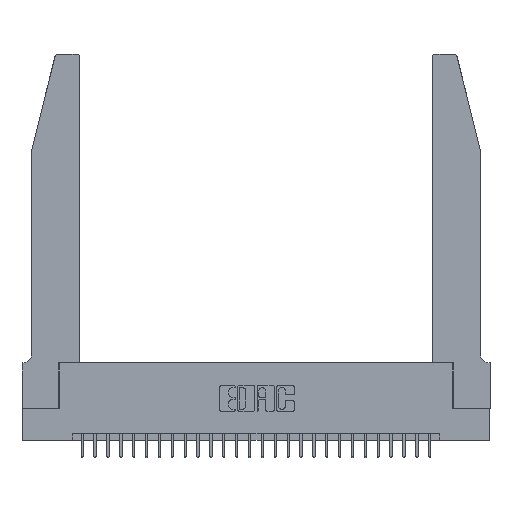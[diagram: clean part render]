
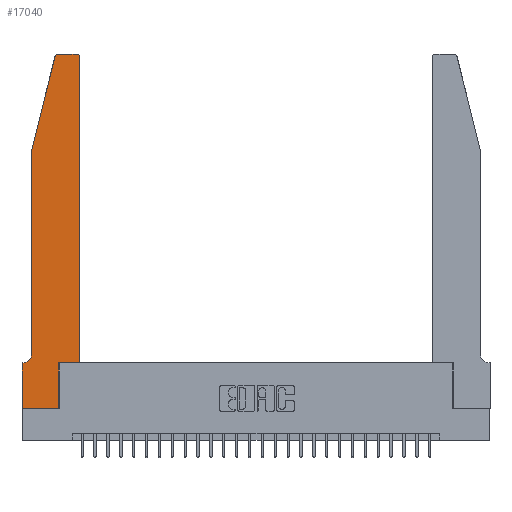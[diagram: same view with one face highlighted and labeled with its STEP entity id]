
A CAD part, top view. The second image highlights one B-rep face of the part: STEP entity #17040.
In plain terms, the highlighted planar face has unit normal (0, 0, 1).
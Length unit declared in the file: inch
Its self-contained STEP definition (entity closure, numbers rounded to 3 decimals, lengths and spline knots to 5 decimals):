
#171 = EDGE_CURVE ( 'NONE', #16835, #24822, #9577, .T. ) ;
#645 = EDGE_CURVE ( 'NONE', #26955, #16835, #19283, .T. ) ;
#752 = LINE ( 'NONE', #22707, #5583 ) ;
#1592 = VERTEX_POINT ( 'NONE', #20082 ) ;
#1924 = CARTESIAN_POINT ( 'NONE',  ( 0., 0.35, 0.37 ) ) ;
#1952 = ORIENTED_EDGE ( 'NONE', *, *, #23661, .T. ) ;
#2432 = ORIENTED_EDGE ( 'NONE', *, *, #6540, .T. ) ;
#2747 = CARTESIAN_POINT ( 'NONE',  ( 0.0755, 2., 0.37 ) ) ;
#3024 = DIRECTION ( 'NONE',  ( 0., 1., 0. ) ) ;
#3047 = LINE ( 'NONE', #7139, #26902 ) ;
#3070 = VECTOR ( 'NONE', #17211, 39.37008 ) ;
#3137 = EDGE_CURVE ( 'NONE', #22423, #17642, #752, .T. ) ;
#3469 = EDGE_LOOP ( 'NONE', ( #27641, #12043, #7407, #23063, #1952, #2432, #8991, #21217, #19030, #14105, #15593, #9170 ) ) ;
#4006 = CARTESIAN_POINT ( 'NONE',  ( 0.284, 2.72, 0.37 ) ) ;
#4182 = VERTEX_POINT ( 'NONE', #27566 ) ;
#4199 = LINE ( 'NONE', #13072, #23433 ) ;
#4328 = EDGE_CURVE ( 'NONE', #17642, #25782, #17723, .T. ) ;
#4674 = CARTESIAN_POINT ( 'NONE',  ( 0., 0., 0.37 ) ) ;
#4693 = CARTESIAN_POINT ( 'NONE',  ( 0.4205, 2.72, 0.37 ) ) ;
#4817 = CARTESIAN_POINT ( 'NONE',  ( 0.0755, 2., 0.37 ) ) ;
#5359 = DIRECTION ( 'NONE',  ( 0., -1., 0. ) ) ;
#5583 = VECTOR ( 'NONE', #18510, 39.37008 ) ;
#5661 = CARTESIAN_POINT ( 'NONE',  ( 0.2865, 0.35, 0.37 ) ) ;
#5664 = VERTEX_POINT ( 'NONE', #7063 ) ;
#6540 = EDGE_CURVE ( 'NONE', #1592, #5664, #3047, .T. ) ;
#7063 = CARTESIAN_POINT ( 'NONE',  ( 0., 0.35, 0.37 ) ) ;
#7139 = CARTESIAN_POINT ( 'NONE',  ( 0.0755, 0.35, 0.37 ) ) ;
#7407 = ORIENTED_EDGE ( 'NONE', *, *, #19415, .T. ) ;
#7457 = CARTESIAN_POINT ( 'NONE',  ( 0.4505, 0.35, 0.37 ) ) ;
#8480 = LINE ( 'NONE', #24032, #3070 ) ;
#8991 = ORIENTED_EDGE ( 'NONE', *, *, #9553, .T. ) ;
#9170 = ORIENTED_EDGE ( 'NONE', *, *, #15286, .T. ) ;
#9180 = DIRECTION ( 'NONE',  ( 0., -1., 0. ) ) ;
#9553 = EDGE_CURVE ( 'NONE', #5664, #13724, #25017, .T. ) ;
#9577 = LINE ( 'NONE', #18894, #24126 ) ;
#10102 = CARTESIAN_POINT ( 'NONE',  ( 0.284, 2.75, 0.37 ) ) ;
#10204 = FACE_OUTER_BOUND ( 'NONE', #3469, .T. ) ;
#10585 = CARTESIAN_POINT ( 'NONE',  ( 0.0755, 0.42, 0.37 ) ) ;
#10708 = DIRECTION ( 'NONE',  ( 1., 0., 0. ) ) ;
#10867 = CARTESIAN_POINT ( 'NONE',  ( 0.0055, 0.42, 0.37 ) ) ;
#10891 = DIRECTION ( 'NONE',  ( 0., 1., 0. ) ) ;
#11003 = VECTOR ( 'NONE', #25019, 39.37008 ) ;
#11468 = CARTESIAN_POINT ( 'NONE',  ( 0., 0., 0.37 ) ) ;
#12043 = ORIENTED_EDGE ( 'NONE', *, *, #4328, .T. ) ;
#12755 = DIRECTION ( 'NONE',  ( 0., 0., -1. ) ) ;
#12779 = VECTOR ( 'NONE', #9180, 39.37008 ) ;
#12880 = DIRECTION ( 'NONE',  ( 0., 0., 1. ) ) ;
#13072 = CARTESIAN_POINT ( 'NONE',  ( 0.2865, 0.35, 0.37 ) ) ;
#13632 = VERTEX_POINT ( 'NONE', #27018 ) ;
#13724 = VERTEX_POINT ( 'NONE', #11468 ) ;
#14105 = ORIENTED_EDGE ( 'NONE', *, *, #645, .T. ) ;
#15121 = CARTESIAN_POINT ( 'NONE',  ( 0.4205, 2.75, 0.37 ) ) ;
#15286 = EDGE_CURVE ( 'NONE', #24822, #22423, #20137, .T. ) ;
#15309 = DIRECTION ( 'NONE',  ( 1., 0., 0. ) ) ;
#15593 = ORIENTED_EDGE ( 'NONE', *, *, #171, .T. ) ;
#16607 = LINE ( 'NONE', #4817, #11003 ) ;
#16835 = VERTEX_POINT ( 'NONE', #7457 ) ;
#16939 = AXIS2_PLACEMENT_3D ( 'NONE', #1924, #19094, #15309 ) ;
#17040 = ADVANCED_FACE ( 'NONE', ( #10204 ), #26178, .T. ) ;
#17211 = DIRECTION ( 'NONE',  ( 1., 0., 0. ) ) ;
#17388 = DIRECTION ( 'NONE',  ( 1., 0., 0. ) ) ;
#17508 = EDGE_CURVE ( 'NONE', #13632, #26955, #4199, .T. ) ;
#17642 = VERTEX_POINT ( 'NONE', #10102 ) ;
#17723 = CIRCLE ( 'NONE', #21889, 0.03 ) ;
#18510 = DIRECTION ( 'NONE',  ( -1., 0., 0. ) ) ;
#18785 = CARTESIAN_POINT ( 'NONE',  ( 0.4505, 2.72, 0.37 ) ) ;
#18894 = CARTESIAN_POINT ( 'NONE',  ( 0.4505, 0.35, 0.37 ) ) ;
#19030 = ORIENTED_EDGE ( 'NONE', *, *, #17508, .T. ) ;
#19094 = DIRECTION ( 'NONE',  ( 0., 0., 1. ) ) ;
#19283 = LINE ( 'NONE', #23491, #23694 ) ;
#19415 = EDGE_CURVE ( 'NONE', #25782, #4182, #16607, .T. ) ;
#20082 = CARTESIAN_POINT ( 'NONE',  ( 0.0055, 0.35, 0.37 ) ) ;
#20137 = CIRCLE ( 'NONE', #20591, 0.03 ) ;
#20466 = DIRECTION ( 'NONE',  ( -1., 0., 0. ) ) ;
#20591 = AXIS2_PLACEMENT_3D ( 'NONE', #4693, #24194, #24330 ) ;
#21217 = ORIENTED_EDGE ( 'NONE', *, *, #25777, .T. ) ;
#21299 = CIRCLE ( 'NONE', #25455, 0.07 ) ;
#21710 = CARTESIAN_POINT ( 'NONE',  ( 0.25487, 2.72718, 0.37 ) ) ;
#21889 = AXIS2_PLACEMENT_3D ( 'NONE', #4006, #12880, #10708 ) ;
#22255 = EDGE_CURVE ( 'NONE', #4182, #26745, #24993, .T. ) ;
#22423 = VERTEX_POINT ( 'NONE', #15121 ) ;
#22707 = CARTESIAN_POINT ( 'NONE',  ( 0.2605, 2.75, 0.37 ) ) ;
#22834 = DIRECTION ( 'NONE',  ( -1., 0., 0. ) ) ;
#23063 = ORIENTED_EDGE ( 'NONE', *, *, #22255, .T. ) ;
#23433 = VECTOR ( 'NONE', #10891, 39.37008 ) ;
#23491 = CARTESIAN_POINT ( 'NONE',  ( 0.4505, 0.35, 0.37 ) ) ;
#23661 = EDGE_CURVE ( 'NONE', #26745, #1592, #21299, .T. ) ;
#23694 = VECTOR ( 'NONE', #17388, 39.37008 ) ;
#24032 = CARTESIAN_POINT ( 'NONE',  ( 0., 0., 0.37 ) ) ;
#24126 = VECTOR ( 'NONE', #3024, 39.37008 ) ;
#24194 = DIRECTION ( 'NONE',  ( 0., 0., 1. ) ) ;
#24330 = DIRECTION ( 'NONE',  ( 1., 0., 0. ) ) ;
#24822 = VERTEX_POINT ( 'NONE', #18785 ) ;
#24993 = LINE ( 'NONE', #2747, #27736 ) ;
#25017 = LINE ( 'NONE', #4674, #12779 ) ;
#25019 = DIRECTION ( 'NONE',  ( -0.239, -0.971, 0. ) ) ;
#25455 = AXIS2_PLACEMENT_3D ( 'NONE', #10867, #12755, #20466 ) ;
#25777 = EDGE_CURVE ( 'NONE', #13724, #13632, #8480, .T. ) ;
#25782 = VERTEX_POINT ( 'NONE', #21710 ) ;
#26178 = PLANE ( 'NONE',  #16939 ) ;
#26745 = VERTEX_POINT ( 'NONE', #10585 ) ;
#26902 = VECTOR ( 'NONE', #22834, 39.37008 ) ;
#26955 = VERTEX_POINT ( 'NONE', #5661 ) ;
#27018 = CARTESIAN_POINT ( 'NONE',  ( 0.2865, 0., 0.37 ) ) ;
#27566 = CARTESIAN_POINT ( 'NONE',  ( 0.0755, 2., 0.37 ) ) ;
#27641 = ORIENTED_EDGE ( 'NONE', *, *, #3137, .T. ) ;
#27736 = VECTOR ( 'NONE', #5359, 39.37008 ) ;
